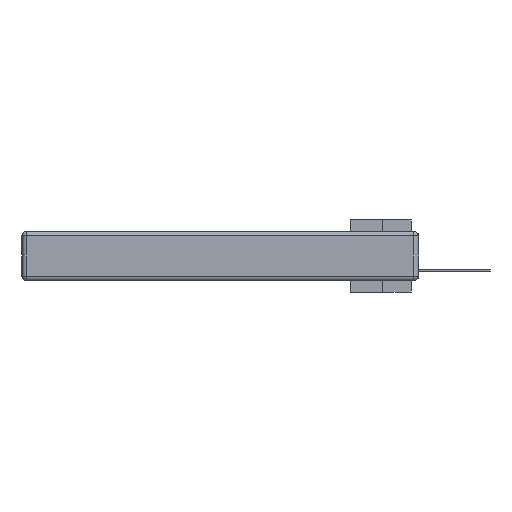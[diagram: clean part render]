
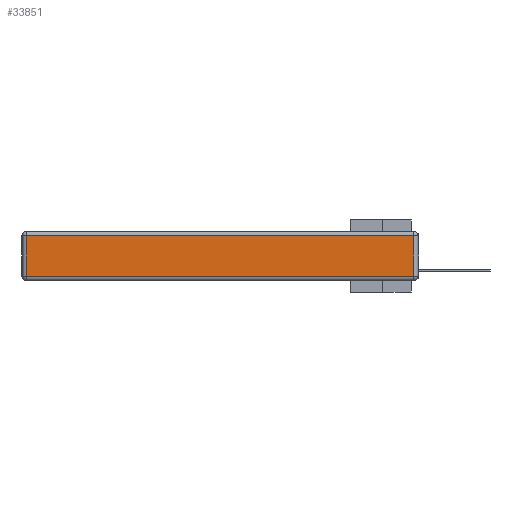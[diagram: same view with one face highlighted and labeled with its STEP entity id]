
A CAD part, left-side view. The second image highlights one B-rep face of the part: STEP entity #33851.
In plain terms, the highlighted planar face has unit normal (-1, 0, 0).
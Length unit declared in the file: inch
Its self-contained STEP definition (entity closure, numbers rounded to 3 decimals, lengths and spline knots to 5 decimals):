
#2390 = LINE ( 'NONE', #20387, #32733 ) ;
#2796 = FACE_OUTER_BOUND ( 'NONE', #2963, .T. ) ;
#2963 = EDGE_LOOP ( 'NONE', ( #35622, #11326, #19170, #21617 ) ) ;
#3234 = VERTEX_POINT ( 'NONE', #3493 ) ;
#3493 = CARTESIAN_POINT ( 'NONE',  ( 0., 2.72, -0.313 ) ) ;
#4525 = AXIS2_PLACEMENT_3D ( 'NONE', #29261, #38283, #15108 ) ;
#5493 = LINE ( 'NONE', #35683, #37561 ) ;
#5712 = PLANE ( 'NONE',  #4525 ) ;
#6141 = VERTEX_POINT ( 'NONE', #27668 ) ;
#7343 = VERTEX_POINT ( 'NONE', #20268 ) ;
#9037 = VECTOR ( 'NONE', #10351, 39.37008 ) ;
#10351 = DIRECTION ( 'NONE',  ( 0., 1., 0. ) ) ;
#11326 = ORIENTED_EDGE ( 'NONE', *, *, #35643, .T. ) ;
#15108 = DIRECTION ( 'NONE',  ( 0., 0., 1. ) ) ;
#15865 = EDGE_CURVE ( 'NONE', #3234, #30490, #20846, .T. ) ;
#18014 = DIRECTION ( 'NONE',  ( 0., 0., 1. ) ) ;
#19169 = LINE ( 'NONE', #22086, #9037 ) ;
#19170 = ORIENTED_EDGE ( 'NONE', *, *, #35919, .T. ) ;
#20268 = CARTESIAN_POINT ( 'NONE',  ( 0., 0.03, -0.03 ) ) ;
#20387 = CARTESIAN_POINT ( 'NONE',  ( 0., 0.03, -0.343 ) ) ;
#20846 = LINE ( 'NONE', #35978, #31484 ) ;
#21617 = ORIENTED_EDGE ( 'NONE', *, *, #31184, .T. ) ;
#22086 = CARTESIAN_POINT ( 'NONE',  ( 0., 2.75, -0.03 ) ) ;
#27668 = CARTESIAN_POINT ( 'NONE',  ( 0., 2.72, -0.03 ) ) ;
#29261 = CARTESIAN_POINT ( 'NONE',  ( 0., 0., -0.343 ) ) ;
#29319 = DIRECTION ( 'NONE',  ( 0., -1., 0. ) ) ;
#30490 = VERTEX_POINT ( 'NONE', #36735 ) ;
#31184 = EDGE_CURVE ( 'NONE', #6141, #3234, #5493, .T. ) ;
#31484 = VECTOR ( 'NONE', #29319, 39.37008 ) ;
#32733 = VECTOR ( 'NONE', #18014, 39.37008 ) ;
#33851 = ADVANCED_FACE ( 'NONE', ( #2796 ), #5712, .T. ) ;
#35085 = DIRECTION ( 'NONE',  ( 0., 0., -1. ) ) ;
#35622 = ORIENTED_EDGE ( 'NONE', *, *, #15865, .T. ) ;
#35643 = EDGE_CURVE ( 'NONE', #30490, #7343, #2390, .T. ) ;
#35683 = CARTESIAN_POINT ( 'NONE',  ( 0., 2.72, -0.343 ) ) ;
#35919 = EDGE_CURVE ( 'NONE', #7343, #6141, #19169, .T. ) ;
#35978 = CARTESIAN_POINT ( 'NONE',  ( 0., 0., -0.313 ) ) ;
#36735 = CARTESIAN_POINT ( 'NONE',  ( 0., 0.03, -0.313 ) ) ;
#37561 = VECTOR ( 'NONE', #35085, 39.37008 ) ;
#38283 = DIRECTION ( 'NONE',  ( -1., 0., 0. ) ) ;
